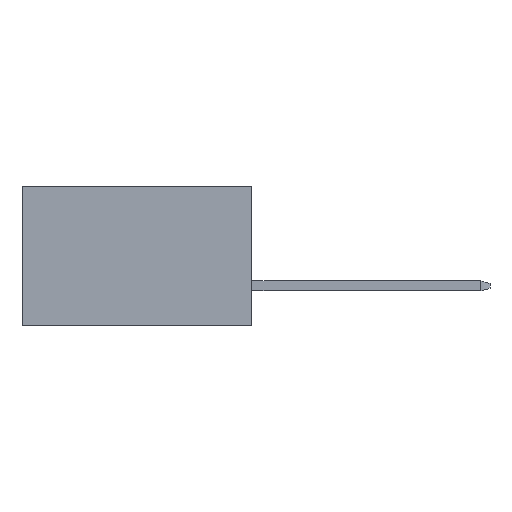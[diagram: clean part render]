
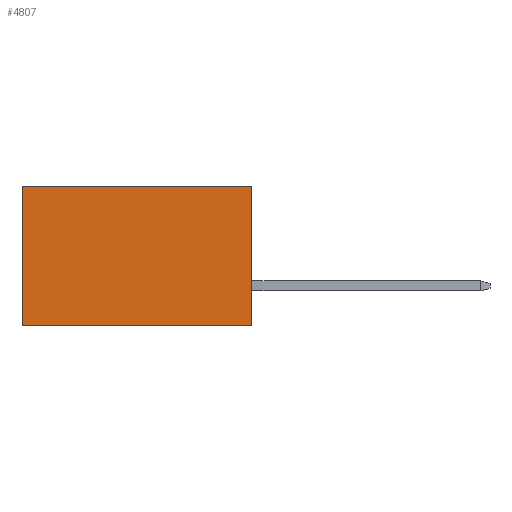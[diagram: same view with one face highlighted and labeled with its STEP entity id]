
A CAD part, left-side view. The second image highlights one B-rep face of the part: STEP entity #4807.
In plain terms, the highlighted planar face has unit normal (-1, 0, 0).
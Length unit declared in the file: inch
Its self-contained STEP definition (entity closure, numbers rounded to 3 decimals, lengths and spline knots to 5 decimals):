
#484 = PLANE ( 'NONE',  #8356 ) ;
#625 = CARTESIAN_POINT ( 'NONE',  ( 0.3205, 0.72, 0. ) ) ;
#973 = DIRECTION ( 'NONE',  ( 0., 0., -1. ) ) ;
#1142 = CARTESIAN_POINT ( 'NONE',  ( 0.3205, 0., -0.437 ) ) ;
#1200 = ORIENTED_EDGE ( 'NONE', *, *, #4578, .F. ) ;
#1228 = LINE ( 'NONE', #1142, #6844 ) ;
#1579 = VERTEX_POINT ( 'NONE', #625 ) ;
#2262 = DIRECTION ( 'NONE',  ( 0., 0., -1. ) ) ;
#2403 = DIRECTION ( 'NONE',  ( 1., 0., 0. ) ) ;
#2415 = VERTEX_POINT ( 'NONE', #7445 ) ;
#2785 = EDGE_CURVE ( 'NONE', #2415, #1579, #6618, .T. ) ;
#2873 = CARTESIAN_POINT ( 'NONE',  ( 0.3205, 0.72, -0.437 ) ) ;
#3113 = EDGE_CURVE ( 'NONE', #3847, #8385, #1228, .T. ) ;
#3288 = VECTOR ( 'NONE', #7304, 39.37008 ) ;
#3601 = EDGE_LOOP ( 'NONE', ( #7239, #4322, #1200, #8042 ) ) ;
#3847 = VERTEX_POINT ( 'NONE', #4133 ) ;
#4133 = CARTESIAN_POINT ( 'NONE',  ( 0.3205, 0., -0.437 ) ) ;
#4179 = LINE ( 'NONE', #2873, #6332 ) ;
#4322 = ORIENTED_EDGE ( 'NONE', *, *, #3113, .F. ) ;
#4578 = EDGE_CURVE ( 'NONE', #2415, #3847, #6128, .T. ) ;
#4807 = ADVANCED_FACE ( 'NONE', ( #6428 ), #484, .F. ) ;
#5380 = DIRECTION ( 'NONE',  ( 0., 0., -1. ) ) ;
#5403 = CARTESIAN_POINT ( 'NONE',  ( 0.3205, 0., 0. ) ) ;
#5659 = CARTESIAN_POINT ( 'NONE',  ( 0.3205, 0., -0.437 ) ) ;
#5911 = CARTESIAN_POINT ( 'NONE',  ( 0.3205, 0.72, -0.437 ) ) ;
#6128 = LINE ( 'NONE', #5659, #7939 ) ;
#6332 = VECTOR ( 'NONE', #5380, 39.37008 ) ;
#6428 = FACE_OUTER_BOUND ( 'NONE', #3601, .T. ) ;
#6618 = LINE ( 'NONE', #5403, #3288 ) ;
#6844 = VECTOR ( 'NONE', #8423, 39.37008 ) ;
#7239 = ORIENTED_EDGE ( 'NONE', *, *, #7649, .T. ) ;
#7304 = DIRECTION ( 'NONE',  ( 0., 1., 0. ) ) ;
#7445 = CARTESIAN_POINT ( 'NONE',  ( 0.3205, 0., 0. ) ) ;
#7649 = EDGE_CURVE ( 'NONE', #1579, #8385, #4179, .T. ) ;
#7806 = CARTESIAN_POINT ( 'NONE',  ( 0.3205, 0., -0.437 ) ) ;
#7939 = VECTOR ( 'NONE', #973, 39.37008 ) ;
#8042 = ORIENTED_EDGE ( 'NONE', *, *, #2785, .T. ) ;
#8356 = AXIS2_PLACEMENT_3D ( 'NONE', #7806, #2403, #2262 ) ;
#8385 = VERTEX_POINT ( 'NONE', #5911 ) ;
#8423 = DIRECTION ( 'NONE',  ( 0., 1., 0. ) ) ;
